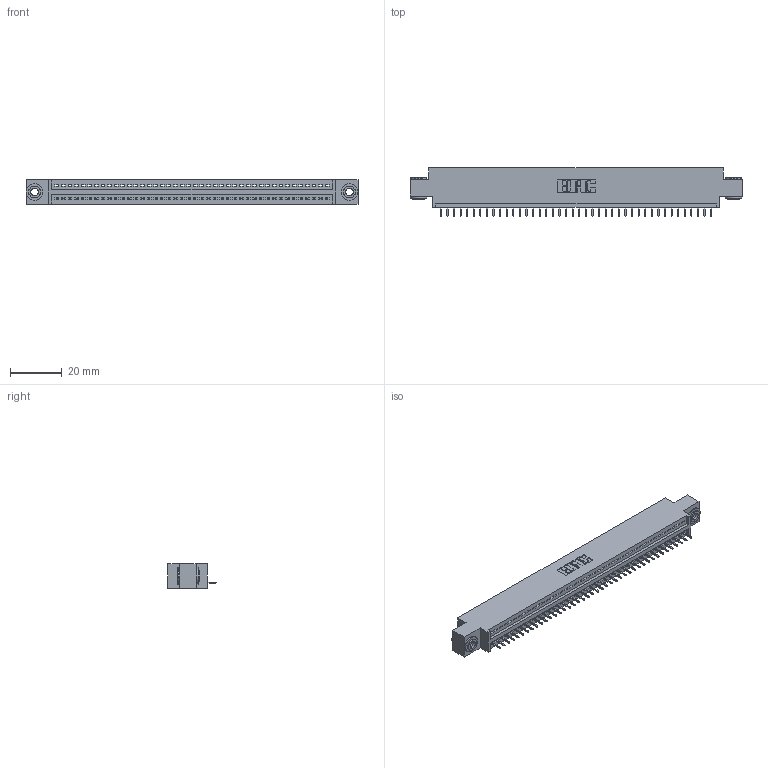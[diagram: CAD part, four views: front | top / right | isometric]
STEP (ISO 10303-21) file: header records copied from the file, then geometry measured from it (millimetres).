
FILE_DESCRIPTION (( 'STEP AP203' ), '1' );
FILE_NAME ('895-042-525-603.STEP', '2020-09-27T01:50:48', ( '' ), ( '' ), 'SwSTEP 2.0', 'SolidWorks 2020', '' );
FILE_SCHEMA (( 'CONFIG_CONTROL_DESIGN' ));
Length unit declared in the file: inch
Products named in the file (4): 845 Part_0.170 Offset - 0.156 Dia-TH; 345-292-001_345-293-125; 345-250-002_345-250-002-102; 895-042-525-603
Assembly tree (45 placements, depth 2):
  895-042-525-603
    845 Part_0.170 Offset - 0.156 Dia-TH
    345-292-001_345-293-125  x42
    345-250-002_345-250-002-102  x2
Bounding box: 127.89 x 18.72 x 9.4 mm (x, y, z)
Volume: 11881.6 mm3; surface area: 15558.7 mm2
Topology: 45 solids, 45 shells, 2772 faces, 7989 edges, 5154 vertices
Faces by surface type: plane 2026, cylinder 738, cone 8
Entity records: 32466 total; most frequent: CARTESIAN_POINT 5601, ORIENTED_EDGE 5570, DIRECTION 4923, EDGE_CURVE 2785, LINE 2465, VECTOR 2465, VERTEX_POINT 1850, AXIS2_PLACEMENT_3D 1229
